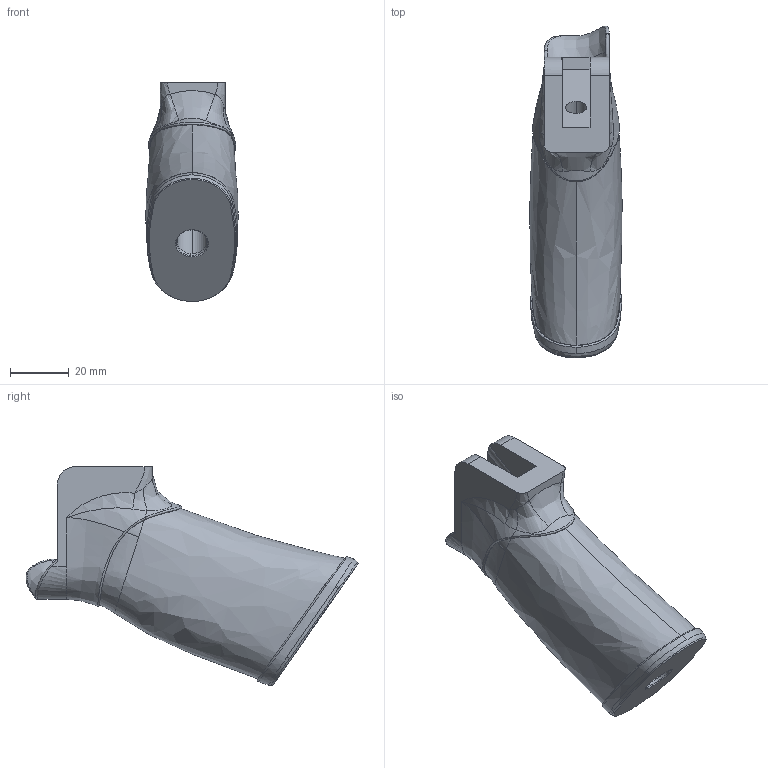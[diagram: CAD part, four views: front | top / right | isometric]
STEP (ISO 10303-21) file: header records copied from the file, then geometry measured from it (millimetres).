
FILE_DESCRIPTION (( 'STEP AP203' ), '1' );
FILE_NAME ('Grip V3.1 Legacy TR.STEP', '2022-05-14T17:17:50', ( '' ), ( '' ), 'SwSTEP 2.0', 'SolidWorks 2021', '' );
FILE_SCHEMA (( 'CONFIG_CONTROL_DESIGN' ));
Length unit declared in the file: inch
Products named in the file (1): Grip V3.1 Legacy TR
Bounding box: 31.48 x 113.41 x 74.79 mm (x, y, z)
Volume: 98009 mm3; surface area: 18361.6 mm2
Topology: 1 solids, 1 shells, 81 faces, 222 edges, 141 vertices
Faces by surface type: bspline 53, plane 14, cylinder 12, torus 2
Entity records: 22632 total; most frequent: CARTESIAN_POINT 20986, ORIENTED_EDGE 434, EDGE_CURVE 217, DIRECTION 155, VERTEX_POINT 141, B_SPLINE_CURVE_WITH_KNOTS 139, EDGE_LOOP 86, ADVANCED_FACE 81
